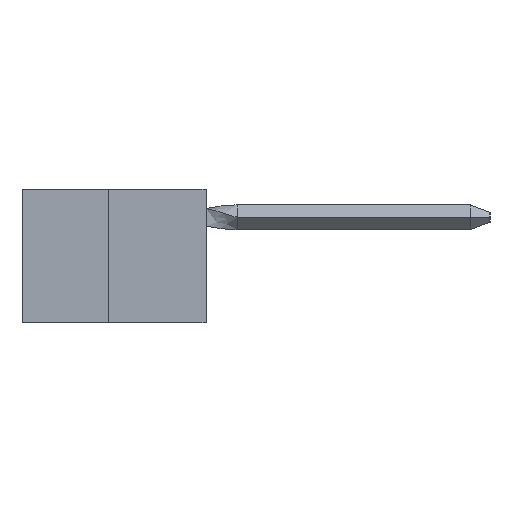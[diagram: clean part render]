
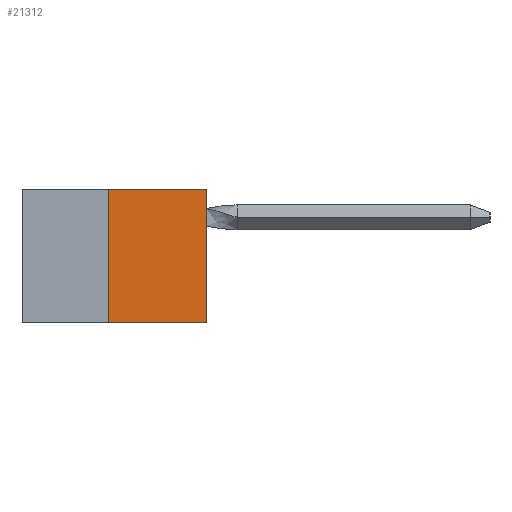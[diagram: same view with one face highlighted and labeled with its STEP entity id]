
A CAD part, left-side view. The second image highlights one B-rep face of the part: STEP entity #21312.
In plain terms, the highlighted planar face has unit normal (-1, 0, 0).
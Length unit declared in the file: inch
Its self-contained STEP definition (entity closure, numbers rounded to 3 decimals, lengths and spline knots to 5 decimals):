
#1282 = ORIENTED_EDGE ( 'NONE', *, *, #2027, .T. ) ;
#1405 = DIRECTION ( 'NONE',  ( 0., -1., 0. ) ) ;
#2027 = EDGE_CURVE ( 'NONE', #18828, #21596, #20207, .T. ) ;
#2071 = CARTESIAN_POINT ( 'NONE',  ( 0., 0.25, 0. ) ) ;
#2160 = CARTESIAN_POINT ( 'NONE',  ( 0., 0.473, -0.343 ) ) ;
#3086 = AXIS2_PLACEMENT_3D ( 'NONE', #22337, #22439, #17238 ) ;
#3548 = CARTESIAN_POINT ( 'NONE',  ( 0., 0., -0.343 ) ) ;
#4282 = VECTOR ( 'NONE', #1405, 39.37008 ) ;
#4928 = EDGE_CURVE ( 'NONE', #17369, #18828, #17367, .T. ) ;
#5043 = LINE ( 'NONE', #13812, #4282 ) ;
#7150 = ORIENTED_EDGE ( 'NONE', *, *, #10472, .F. ) ;
#9401 = CARTESIAN_POINT ( 'NONE',  ( 0., 0.25, -0.343 ) ) ;
#9424 = VECTOR ( 'NONE', #19493, 39.37008 ) ;
#9702 = ORIENTED_EDGE ( 'NONE', *, *, #20277, .F. ) ;
#10472 = EDGE_CURVE ( 'NONE', #29965, #21596, #5043, .T. ) ;
#11649 = CARTESIAN_POINT ( 'NONE',  ( 0., 0., 0. ) ) ;
#12049 = DIRECTION ( 'NONE',  ( 0., 0., 1. ) ) ;
#12795 = VECTOR ( 'NONE', #21825, 39.37008 ) ;
#13812 = CARTESIAN_POINT ( 'NONE',  ( 0., 0.473, 0. ) ) ;
#14278 = EDGE_LOOP ( 'NONE', ( #7150, #9702, #27280, #1282 ) ) ;
#14784 = PLANE ( 'NONE',  #3086 ) ;
#15276 = VECTOR ( 'NONE', #12049, 39.37008 ) ;
#17238 = DIRECTION ( 'NONE',  ( 0., 0., -1. ) ) ;
#17367 = LINE ( 'NONE', #2160, #12795 ) ;
#17369 = VERTEX_POINT ( 'NONE', #9401 ) ;
#18675 = FACE_OUTER_BOUND ( 'NONE', #14278, .T. ) ;
#18828 = VERTEX_POINT ( 'NONE', #3548 ) ;
#19493 = DIRECTION ( 'NONE',  ( 0., 0., 1. ) ) ;
#20207 = LINE ( 'NONE', #31548, #15276 ) ;
#20277 = EDGE_CURVE ( 'NONE', #17369, #29965, #28093, .T. ) ;
#21312 = ADVANCED_FACE ( 'NONE', ( #18675 ), #14784, .F. ) ;
#21596 = VERTEX_POINT ( 'NONE', #11649 ) ;
#21825 = DIRECTION ( 'NONE',  ( 0., -1., 0. ) ) ;
#22337 = CARTESIAN_POINT ( 'NONE',  ( 0., 0.473, 0. ) ) ;
#22439 = DIRECTION ( 'NONE',  ( 1., 0., 0. ) ) ;
#27280 = ORIENTED_EDGE ( 'NONE', *, *, #4928, .T. ) ;
#28093 = LINE ( 'NONE', #31530, #9424 ) ;
#29965 = VERTEX_POINT ( 'NONE', #2071 ) ;
#31530 = CARTESIAN_POINT ( 'NONE',  ( 0., 0.25, 0. ) ) ;
#31548 = CARTESIAN_POINT ( 'NONE',  ( 0., 0., 0. ) ) ;
